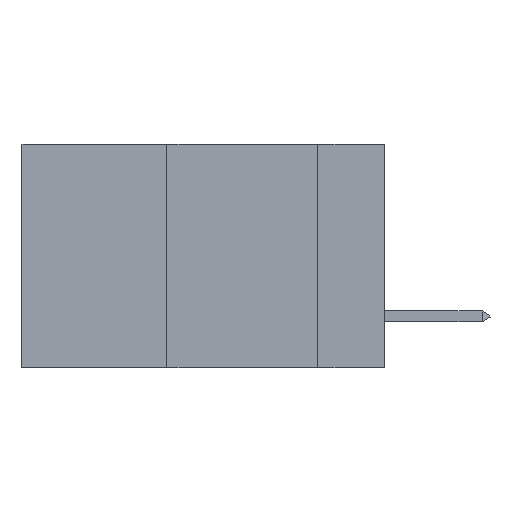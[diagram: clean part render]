
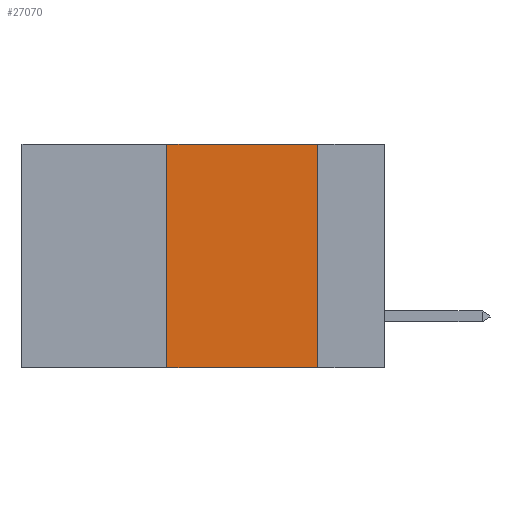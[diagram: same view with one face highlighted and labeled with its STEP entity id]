
A CAD part, left-side view. The second image highlights one B-rep face of the part: STEP entity #27070.
In plain terms, the highlighted planar face has unit normal (-1, 0, 0).
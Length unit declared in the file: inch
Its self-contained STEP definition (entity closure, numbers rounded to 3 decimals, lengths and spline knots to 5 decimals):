
#755 = DIRECTION ( 'NONE',  ( 0., 0., 1. ) ) ;
#838 = EDGE_CURVE ( 'NONE', #24294, #3959, #37380, .T. ) ;
#1025 = VECTOR ( 'NONE', #755, 39.37008 ) ;
#2564 = ORIENTED_EDGE ( 'NONE', *, *, #17233, .F. ) ;
#2655 = CARTESIAN_POINT ( 'NONE',  ( 0., 0.36, -0.37 ) ) ;
#3185 = VERTEX_POINT ( 'NONE', #2655 ) ;
#3472 = CARTESIAN_POINT ( 'NONE',  ( 0., 0.11, 0. ) ) ;
#3629 = CARTESIAN_POINT ( 'NONE',  ( 0., 0.11, -0.37 ) ) ;
#3959 = VERTEX_POINT ( 'NONE', #3472 ) ;
#3974 = VERTEX_POINT ( 'NONE', #3629 ) ;
#5514 = DIRECTION ( 'NONE',  ( 0., 0., -1. ) ) ;
#6352 = VECTOR ( 'NONE', #15907, 39.37008 ) ;
#8031 = CARTESIAN_POINT ( 'NONE',  ( 0., 0.6, 0. ) ) ;
#8999 = VECTOR ( 'NONE', #45509, 39.37008 ) ;
#13920 = EDGE_CURVE ( 'NONE', #3959, #3974, #14902, .T. ) ;
#14902 = LINE ( 'NONE', #28870, #45857 ) ;
#14956 = DIRECTION ( 'NONE',  ( 1., 0., 0. ) ) ;
#15907 = DIRECTION ( 'NONE',  ( 0., -1., 0. ) ) ;
#17233 = EDGE_CURVE ( 'NONE', #3185, #24294, #32101, .T. ) ;
#23392 = ORIENTED_EDGE ( 'NONE', *, *, #13920, .F. ) ;
#24274 = FACE_OUTER_BOUND ( 'NONE', #27869, .T. ) ;
#24294 = VERTEX_POINT ( 'NONE', #35363 ) ;
#26516 = PLANE ( 'NONE',  #30995 ) ;
#27070 = ADVANCED_FACE ( 'NONE', ( #24274 ), #26516, .F. ) ;
#27869 = EDGE_LOOP ( 'NONE', ( #23392, #37279, #2564, #28803 ) ) ;
#28803 = ORIENTED_EDGE ( 'NONE', *, *, #49714, .T. ) ;
#28870 = CARTESIAN_POINT ( 'NONE',  ( 0., 0.11, 0. ) ) ;
#30995 = AXIS2_PLACEMENT_3D ( 'NONE', #49684, #14956, #42060 ) ;
#32101 = LINE ( 'NONE', #47320, #1025 ) ;
#35363 = CARTESIAN_POINT ( 'NONE',  ( 0., 0.36, 0. ) ) ;
#37279 = ORIENTED_EDGE ( 'NONE', *, *, #838, .F. ) ;
#37380 = LINE ( 'NONE', #8031, #6352 ) ;
#39993 = LINE ( 'NONE', #41607, #8999 ) ;
#41607 = CARTESIAN_POINT ( 'NONE',  ( 0., 0.6, -0.37 ) ) ;
#42060 = DIRECTION ( 'NONE',  ( 0., 0., -1. ) ) ;
#45509 = DIRECTION ( 'NONE',  ( 0., -1., 0. ) ) ;
#45857 = VECTOR ( 'NONE', #5514, 39.37008 ) ;
#47320 = CARTESIAN_POINT ( 'NONE',  ( 0., 0.36, 0. ) ) ;
#49684 = CARTESIAN_POINT ( 'NONE',  ( 0., 0.6, 0. ) ) ;
#49714 = EDGE_CURVE ( 'NONE', #3185, #3974, #39993, .T. ) ;
